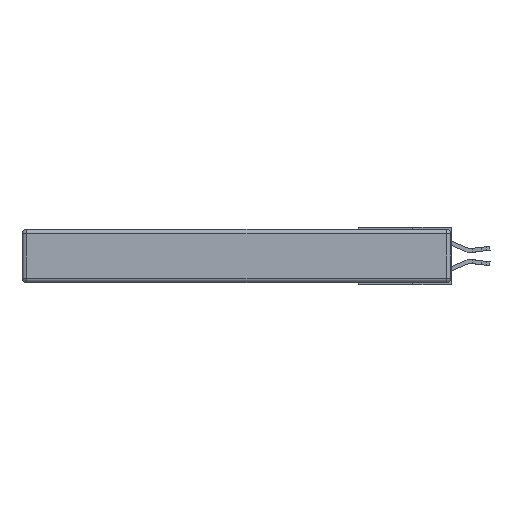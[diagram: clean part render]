
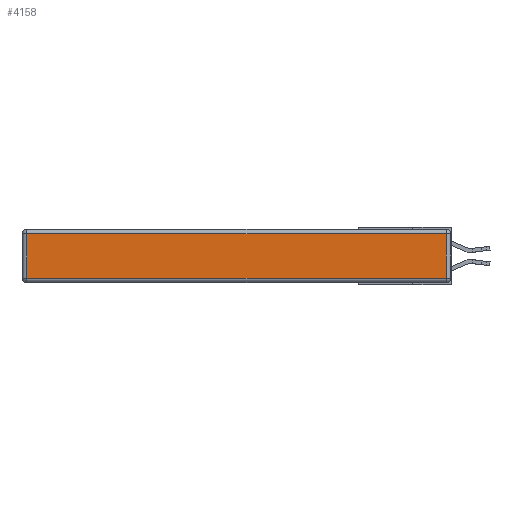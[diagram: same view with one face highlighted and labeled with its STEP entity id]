
A CAD part, left-side view. The second image highlights one B-rep face of the part: STEP entity #4158.
In plain terms, the highlighted planar face has unit normal (-1, 0, 0).
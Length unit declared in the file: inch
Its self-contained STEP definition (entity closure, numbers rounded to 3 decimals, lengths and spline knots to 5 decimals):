
#2018 = CARTESIAN_POINT ( 'NONE',  ( 0., 2.72, -0.03 ) ) ;
#3890 = CARTESIAN_POINT ( 'NONE',  ( 0., 0.03, -0.03 ) ) ;
#3927 = CARTESIAN_POINT ( 'NONE',  ( 0., 2.72, -0.313 ) ) ;
#4158 = ADVANCED_FACE ( 'NONE', ( #22295 ), #15289, .T. ) ;
#4769 = VECTOR ( 'NONE', #9189, 39.37008 ) ;
#5695 = EDGE_CURVE ( 'NONE', #13982, #22635, #6796, .T. ) ;
#5907 = ORIENTED_EDGE ( 'NONE', *, *, #5695, .T. ) ;
#6796 = LINE ( 'NONE', #7029, #4769 ) ;
#7029 = CARTESIAN_POINT ( 'NONE',  ( 0., 0.03, -0.343 ) ) ;
#7141 = VERTEX_POINT ( 'NONE', #3927 ) ;
#7685 = VECTOR ( 'NONE', #11223, 39.37008 ) ;
#9189 = DIRECTION ( 'NONE',  ( 0., 0., 1. ) ) ;
#9901 = CARTESIAN_POINT ( 'NONE',  ( 0., 0., -0.313 ) ) ;
#10557 = VECTOR ( 'NONE', #19177, 39.37008 ) ;
#10635 = CARTESIAN_POINT ( 'NONE',  ( 0., 0., -0.343 ) ) ;
#11223 = DIRECTION ( 'NONE',  ( 0., 0., -1. ) ) ;
#11807 = CARTESIAN_POINT ( 'NONE',  ( 0., 0.03, -0.313 ) ) ;
#12755 = EDGE_LOOP ( 'NONE', ( #17416, #5907, #25273, #13712 ) ) ;
#13076 = DIRECTION ( 'NONE',  ( 0., 0., 1. ) ) ;
#13143 = VERTEX_POINT ( 'NONE', #2018 ) ;
#13458 = EDGE_CURVE ( 'NONE', #13143, #7141, #25187, .T. ) ;
#13712 = ORIENTED_EDGE ( 'NONE', *, *, #13458, .T. ) ;
#13982 = VERTEX_POINT ( 'NONE', #11807 ) ;
#15289 = PLANE ( 'NONE',  #17699 ) ;
#15544 = LINE ( 'NONE', #9901, #18277 ) ;
#16458 = DIRECTION ( 'NONE',  ( 0., -1., 0. ) ) ;
#17416 = ORIENTED_EDGE ( 'NONE', *, *, #26027, .T. ) ;
#17699 = AXIS2_PLACEMENT_3D ( 'NONE', #10635, #23895, #13076 ) ;
#18277 = VECTOR ( 'NONE', #16458, 39.37008 ) ;
#19177 = DIRECTION ( 'NONE',  ( 0., 1., 0. ) ) ;
#22295 = FACE_OUTER_BOUND ( 'NONE', #12755, .T. ) ;
#22635 = VERTEX_POINT ( 'NONE', #3890 ) ;
#23895 = DIRECTION ( 'NONE',  ( -1., 0., 0. ) ) ;
#24118 = CARTESIAN_POINT ( 'NONE',  ( 0., 2.72, -0.343 ) ) ;
#25028 = LINE ( 'NONE', #25674, #10557 ) ;
#25187 = LINE ( 'NONE', #24118, #7685 ) ;
#25273 = ORIENTED_EDGE ( 'NONE', *, *, #26064, .T. ) ;
#25674 = CARTESIAN_POINT ( 'NONE',  ( 0., 2.75, -0.03 ) ) ;
#26027 = EDGE_CURVE ( 'NONE', #7141, #13982, #15544, .T. ) ;
#26064 = EDGE_CURVE ( 'NONE', #22635, #13143, #25028, .T. ) ;
